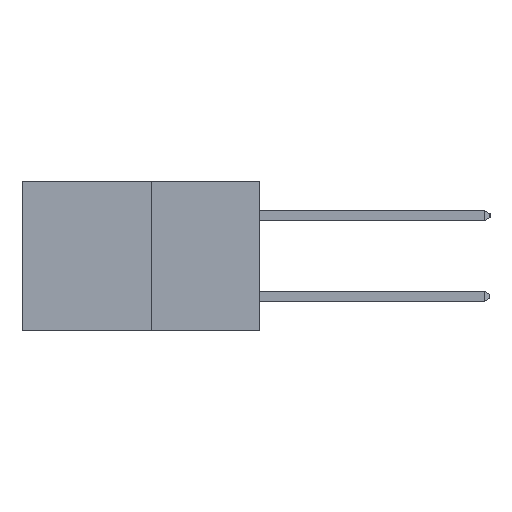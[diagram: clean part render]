
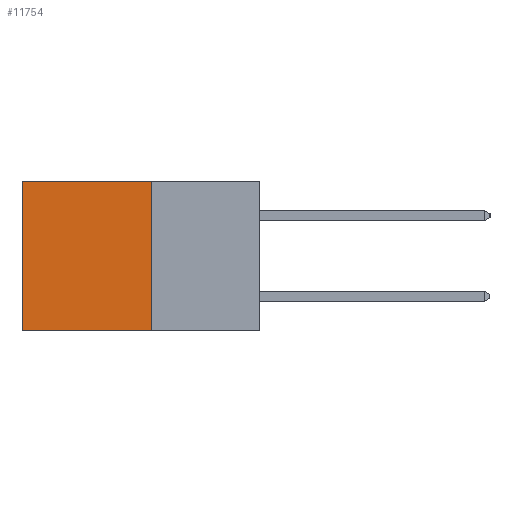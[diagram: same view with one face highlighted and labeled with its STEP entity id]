
A CAD part, left-side view. The second image highlights one B-rep face of the part: STEP entity #11754.
In plain terms, the highlighted planar face has unit normal (-1, 0, 0).
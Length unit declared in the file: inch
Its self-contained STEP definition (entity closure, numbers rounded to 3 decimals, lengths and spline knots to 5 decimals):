
#40 = LINE ( 'NONE', #21212, #8374 ) ;
#348 = ORIENTED_EDGE ( 'NONE', *, *, #4795, .F. ) ;
#796 = CARTESIAN_POINT ( 'NONE',  ( 0.277, 0.27, 0. ) ) ;
#928 = VERTEX_POINT ( 'NONE', #8813 ) ;
#1169 = EDGE_CURVE ( 'NONE', #928, #18880, #10268, .T. ) ;
#1300 = AXIS2_PLACEMENT_3D ( 'NONE', #4760, #16274, #6423 ) ;
#1592 = LINE ( 'NONE', #17791, #18633 ) ;
#3172 = EDGE_LOOP ( 'NONE', ( #21184, #13049, #348, #4845 ) ) ;
#3239 = CARTESIAN_POINT ( 'NONE',  ( 0.277, 0.59, -0.37 ) ) ;
#4760 = CARTESIAN_POINT ( 'NONE',  ( 0.277, 0.27, -0.37 ) ) ;
#4795 = EDGE_CURVE ( 'NONE', #16596, #928, #1592, .T. ) ;
#4845 = ORIENTED_EDGE ( 'NONE', *, *, #19840, .T. ) ;
#6137 = FACE_OUTER_BOUND ( 'NONE', #3172, .T. ) ;
#6423 = DIRECTION ( 'NONE',  ( 0., 0., -1. ) ) ;
#8374 = VECTOR ( 'NONE', #19708, 39.37008 ) ;
#8813 = CARTESIAN_POINT ( 'NONE',  ( 0.277, 0.27, -0.37 ) ) ;
#9760 = VECTOR ( 'NONE', #18714, 39.37008 ) ;
#10268 = LINE ( 'NONE', #18605, #9760 ) ;
#11754 = ADVANCED_FACE ( 'NONE', ( #6137 ), #14580, .F. ) ;
#13049 = ORIENTED_EDGE ( 'NONE', *, *, #1169, .F. ) ;
#13968 = CARTESIAN_POINT ( 'NONE',  ( 0.277, 0.59, 0. ) ) ;
#14580 = PLANE ( 'NONE',  #1300 ) ;
#14729 = VERTEX_POINT ( 'NONE', #13968 ) ;
#14907 = CARTESIAN_POINT ( 'NONE',  ( 0.277, 0.59, -0.37 ) ) ;
#15086 = EDGE_CURVE ( 'NONE', #14729, #18880, #20802, .T. ) ;
#16239 = DIRECTION ( 'NONE',  ( 0., 0., -1. ) ) ;
#16274 = DIRECTION ( 'NONE',  ( 1., 0., 0. ) ) ;
#16528 = DIRECTION ( 'NONE',  ( 0., 0., -1. ) ) ;
#16544 = VECTOR ( 'NONE', #16528, 39.37008 ) ;
#16596 = VERTEX_POINT ( 'NONE', #796 ) ;
#17791 = CARTESIAN_POINT ( 'NONE',  ( 0.277, 0.27, -0.37 ) ) ;
#18605 = CARTESIAN_POINT ( 'NONE',  ( 0.277, 0.27, -0.37 ) ) ;
#18633 = VECTOR ( 'NONE', #16239, 39.37008 ) ;
#18714 = DIRECTION ( 'NONE',  ( 0., 1., 0. ) ) ;
#18880 = VERTEX_POINT ( 'NONE', #3239 ) ;
#19708 = DIRECTION ( 'NONE',  ( 0., 1., 0. ) ) ;
#19840 = EDGE_CURVE ( 'NONE', #16596, #14729, #40, .T. ) ;
#20802 = LINE ( 'NONE', #14907, #16544 ) ;
#21184 = ORIENTED_EDGE ( 'NONE', *, *, #15086, .T. ) ;
#21212 = CARTESIAN_POINT ( 'NONE',  ( 0.277, 0.27, 0. ) ) ;
